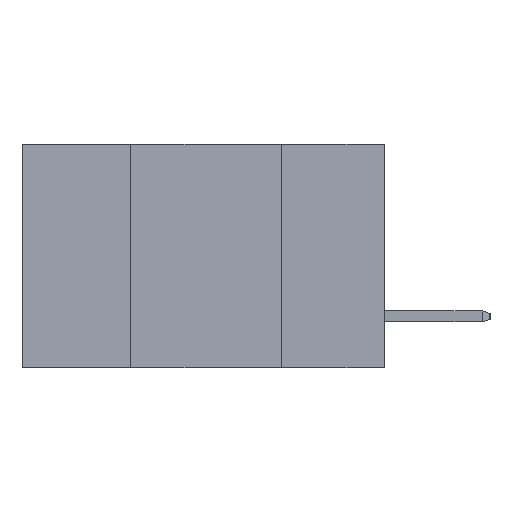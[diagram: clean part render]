
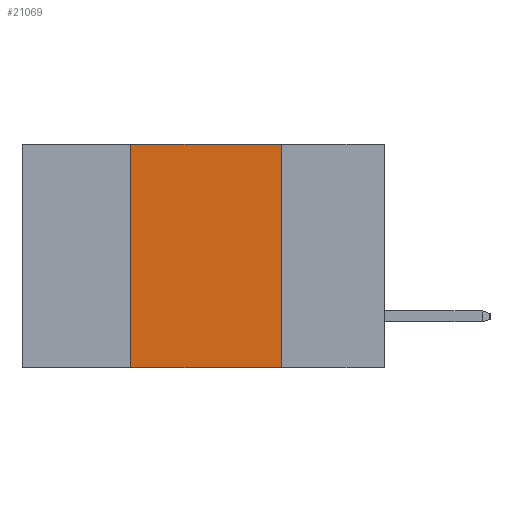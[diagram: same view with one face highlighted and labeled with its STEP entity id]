
A CAD part, left-side view. The second image highlights one B-rep face of the part: STEP entity #21069.
In plain terms, the highlighted planar face has unit normal (-1, 0, 0).
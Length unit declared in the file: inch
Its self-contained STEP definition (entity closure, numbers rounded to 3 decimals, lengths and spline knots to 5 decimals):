
#485 = CARTESIAN_POINT ( 'NONE',  ( 0., 0.42, -0.37 ) ) ;
#735 = DIRECTION ( 'NONE',  ( 0., 0., 1. ) ) ;
#1262 = FACE_OUTER_BOUND ( 'NONE', #18567, .T. ) ;
#2122 = VECTOR ( 'NONE', #23593, 39.37008 ) ;
#2818 = LINE ( 'NONE', #485, #21752 ) ;
#3316 = AXIS2_PLACEMENT_3D ( 'NONE', #17169, #5989, #18975 ) ;
#3433 = CARTESIAN_POINT ( 'NONE',  ( 0., 0.42, 0. ) ) ;
#5286 = VERTEX_POINT ( 'NONE', #3433 ) ;
#5853 = CARTESIAN_POINT ( 'NONE',  ( 0., 0.17, -0.37 ) ) ;
#5989 = DIRECTION ( 'NONE',  ( 1., 0., 0. ) ) ;
#6234 = VERTEX_POINT ( 'NONE', #5853 ) ;
#6318 = ORIENTED_EDGE ( 'NONE', *, *, #10677, .F. ) ;
#6934 = EDGE_CURVE ( 'NONE', #13229, #6234, #13515, .T. ) ;
#8167 = EDGE_CURVE ( 'NONE', #5286, #13229, #14029, .T. ) ;
#10677 = EDGE_CURVE ( 'NONE', #21483, #5286, #2818, .T. ) ;
#11276 = ORIENTED_EDGE ( 'NONE', *, *, #13206, .T. ) ;
#12543 = LINE ( 'NONE', #21842, #2122 ) ;
#12895 = CARTESIAN_POINT ( 'NONE',  ( 0., 0.17, 0. ) ) ;
#13206 = EDGE_CURVE ( 'NONE', #21483, #6234, #12543, .T. ) ;
#13229 = VERTEX_POINT ( 'NONE', #12895 ) ;
#13515 = LINE ( 'NONE', #21547, #17280 ) ;
#14029 = LINE ( 'NONE', #17417, #18909 ) ;
#15102 = ORIENTED_EDGE ( 'NONE', *, *, #6934, .F. ) ;
#16483 = CARTESIAN_POINT ( 'NONE',  ( 0., 0.42, -0.37 ) ) ;
#17077 = PLANE ( 'NONE',  #3316 ) ;
#17162 = DIRECTION ( 'NONE',  ( 0., -1., 0. ) ) ;
#17169 = CARTESIAN_POINT ( 'NONE',  ( 0., 0.6, 0. ) ) ;
#17280 = VECTOR ( 'NONE', #21191, 39.37008 ) ;
#17417 = CARTESIAN_POINT ( 'NONE',  ( 0., 0.6, 0. ) ) ;
#18567 = EDGE_LOOP ( 'NONE', ( #15102, #19923, #6318, #11276 ) ) ;
#18909 = VECTOR ( 'NONE', #17162, 39.37008 ) ;
#18975 = DIRECTION ( 'NONE',  ( 0., 0., -1. ) ) ;
#19923 = ORIENTED_EDGE ( 'NONE', *, *, #8167, .F. ) ;
#21069 = ADVANCED_FACE ( 'NONE', ( #1262 ), #17077, .F. ) ;
#21191 = DIRECTION ( 'NONE',  ( 0., 0., -1. ) ) ;
#21483 = VERTEX_POINT ( 'NONE', #16483 ) ;
#21547 = CARTESIAN_POINT ( 'NONE',  ( 0., 0.17, -0.37 ) ) ;
#21752 = VECTOR ( 'NONE', #735, 39.37008 ) ;
#21842 = CARTESIAN_POINT ( 'NONE',  ( 0., 0.6, -0.37 ) ) ;
#23593 = DIRECTION ( 'NONE',  ( 0., -1., 0. ) ) ;
